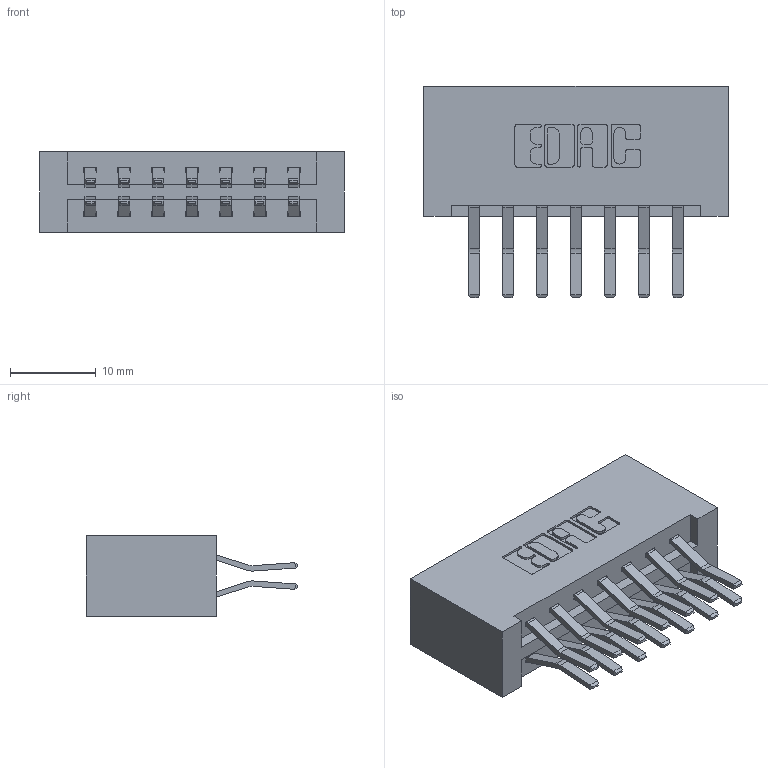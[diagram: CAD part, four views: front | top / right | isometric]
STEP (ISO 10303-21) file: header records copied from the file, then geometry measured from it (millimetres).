
FILE_DESCRIPTION (( 'STEP AP203' ), '1' );
FILE_NAME ('387-014-560-201.STEP', '2018-09-11T06:39:21', ( '' ), ( '' ), 'SwSTEP 2.0', 'SolidWorks 2016', '' );
FILE_SCHEMA (( 'CONFIG_CONTROL_DESIGN' ));
Length unit declared in the file: inch
Products named in the file (3): 337 Part_No Mounting Lugs; 345-292-001_560 Tail; 387-014-560-201
Assembly tree (15 placements, depth 2):
  387-014-560-201
    337 Part_No Mounting Lugs
    345-292-001_560 Tail  x14
Bounding box: 35.61 x 24.78 x 9.4 mm (x, y, z)
Volume: 4139.6 mm3; surface area: 4661.5 mm2
Topology: 15 solids, 15 shells, 890 faces, 2625 edges, 1730 vertices
Faces by surface type: plane 598, cylinder 292
Entity records: 9765 total; most frequent: CARTESIAN_POINT 1674, ORIENTED_EDGE 1610, DIRECTION 1485, EDGE_CURVE 805, LINE 681, VECTOR 681, VERTEX_POINT 534, AXIS2_PLACEMENT_3D 402
